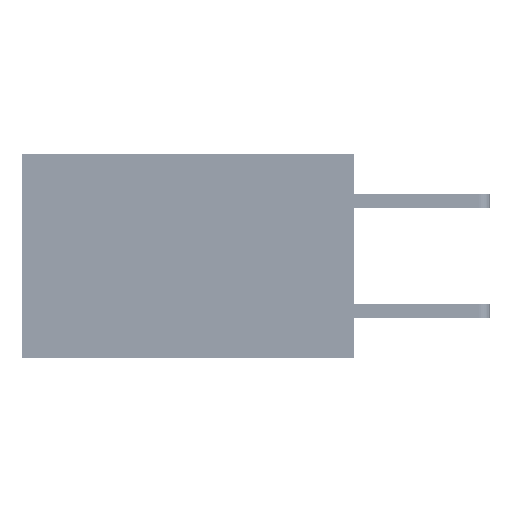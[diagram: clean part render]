
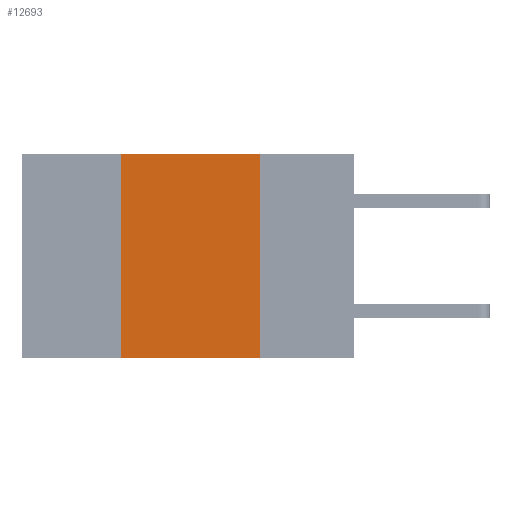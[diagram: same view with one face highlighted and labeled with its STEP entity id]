
A CAD part, left-side view. The second image highlights one B-rep face of the part: STEP entity #12693.
In plain terms, the highlighted planar face has unit normal (-1, 0, 0).
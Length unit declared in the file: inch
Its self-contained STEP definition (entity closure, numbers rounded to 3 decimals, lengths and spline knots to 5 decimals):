
#34 = CARTESIAN_POINT ( 'NONE',  ( 0., 0.42, -0.37 ) ) ;
#2288 = VERTEX_POINT ( 'NONE', #34444 ) ;
#4169 = FACE_OUTER_BOUND ( 'NONE', #43393, .T. ) ;
#5429 = PLANE ( 'NONE',  #22967 ) ;
#5581 = EDGE_CURVE ( 'NONE', #18745, #12940, #34056, .T. ) ;
#5951 = DIRECTION ( 'NONE',  ( 0., 0., -1. ) ) ;
#6327 = CARTESIAN_POINT ( 'NONE',  ( 0., 0.42, 0. ) ) ;
#6955 = CARTESIAN_POINT ( 'NONE',  ( 0., 0.17, 0. ) ) ;
#9062 = VERTEX_POINT ( 'NONE', #34 ) ;
#9425 = ORIENTED_EDGE ( 'NONE', *, *, #29442, .T. ) ;
#10841 = EDGE_CURVE ( 'NONE', #9062, #18745, #47509, .T. ) ;
#11741 = ORIENTED_EDGE ( 'NONE', *, *, #5581, .F. ) ;
#12693 = ADVANCED_FACE ( 'NONE', ( #4169 ), #5429, .F. ) ;
#12940 = VERTEX_POINT ( 'NONE', #6955 ) ;
#15427 = DIRECTION ( 'NONE',  ( 0., -1., 0. ) ) ;
#17249 = LINE ( 'NONE', #32019, #50714 ) ;
#17561 = CARTESIAN_POINT ( 'NONE',  ( 0., 0.6, 0. ) ) ;
#18745 = VERTEX_POINT ( 'NONE', #6327 ) ;
#20086 = CARTESIAN_POINT ( 'NONE',  ( 0., 0.6, -0.37 ) ) ;
#22967 = AXIS2_PLACEMENT_3D ( 'NONE', #17561, #37197, #5951 ) ;
#23049 = ORIENTED_EDGE ( 'NONE', *, *, #43660, .F. ) ;
#28157 = VECTOR ( 'NONE', #36596, 39.37008 ) ;
#28631 = DIRECTION ( 'NONE',  ( 0., 0., -1. ) ) ;
#29442 = EDGE_CURVE ( 'NONE', #9062, #2288, #43588, .T. ) ;
#32019 = CARTESIAN_POINT ( 'NONE',  ( 0., 0.17, 0. ) ) ;
#34056 = LINE ( 'NONE', #50573, #43203 ) ;
#34444 = CARTESIAN_POINT ( 'NONE',  ( 0., 0.17, -0.37 ) ) ;
#35633 = DIRECTION ( 'NONE',  ( 0., 0., 1. ) ) ;
#36596 = DIRECTION ( 'NONE',  ( 0., -1., 0. ) ) ;
#37197 = DIRECTION ( 'NONE',  ( 1., 0., 0. ) ) ;
#43203 = VECTOR ( 'NONE', #15427, 39.37008 ) ;
#43393 = EDGE_LOOP ( 'NONE', ( #23049, #11741, #47928, #9425 ) ) ;
#43588 = LINE ( 'NONE', #20086, #28157 ) ;
#43660 = EDGE_CURVE ( 'NONE', #12940, #2288, #17249, .T. ) ;
#45873 = VECTOR ( 'NONE', #35633, 39.37008 ) ;
#47253 = CARTESIAN_POINT ( 'NONE',  ( 0., 0.42, 0. ) ) ;
#47509 = LINE ( 'NONE', #47253, #45873 ) ;
#47928 = ORIENTED_EDGE ( 'NONE', *, *, #10841, .F. ) ;
#50573 = CARTESIAN_POINT ( 'NONE',  ( 0., 0.6, 0. ) ) ;
#50714 = VECTOR ( 'NONE', #28631, 39.37008 ) ;
